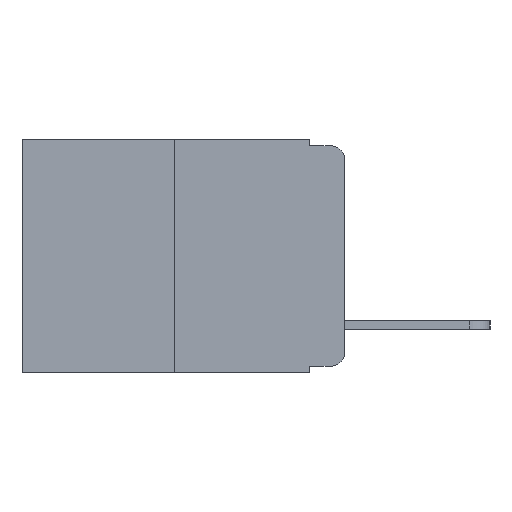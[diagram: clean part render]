
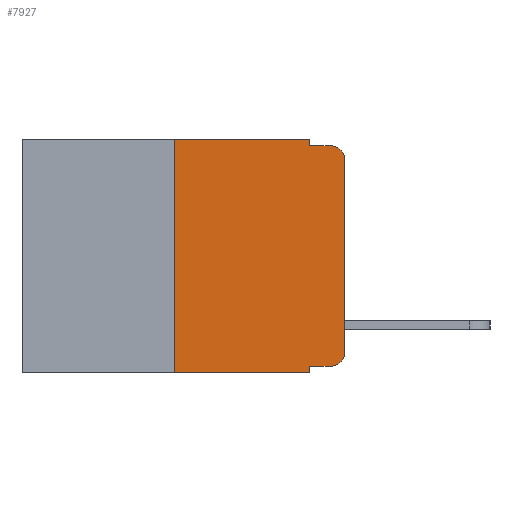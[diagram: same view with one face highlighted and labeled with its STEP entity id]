
A CAD part, left-side view. The second image highlights one B-rep face of the part: STEP entity #7927.
In plain terms, the highlighted planar face has unit normal (-1, 0, 0).
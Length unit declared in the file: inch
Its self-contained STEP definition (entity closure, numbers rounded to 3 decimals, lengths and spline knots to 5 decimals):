
#312 = AXIS2_PLACEMENT_3D ( 'NONE', #5879, #4710, #1290 ) ;
#335 = LINE ( 'NONE', #4685, #9432 ) ;
#344 = ORIENTED_EDGE ( 'NONE', *, *, #2366, .T. ) ;
#508 = DIRECTION ( 'NONE',  ( 0., 0., 1. ) ) ;
#581 = CARTESIAN_POINT ( 'NONE',  ( 0., 0., 0. ) ) ;
#701 = CARTESIAN_POINT ( 'NONE',  ( 0., 0.25, 0. ) ) ;
#743 = ORIENTED_EDGE ( 'NONE', *, *, #3100, .F. ) ;
#872 = ORIENTED_EDGE ( 'NONE', *, *, #5389, .F. ) ;
#877 = VERTEX_POINT ( 'NONE', #701 ) ;
#1074 = VERTEX_POINT ( 'NONE', #11644 ) ;
#1108 = VECTOR ( 'NONE', #1454, 39.37008 ) ;
#1290 = DIRECTION ( 'NONE',  ( 0., 0., -1. ) ) ;
#1291 = ORIENTED_EDGE ( 'NONE', *, *, #4717, .F. ) ;
#1413 = CARTESIAN_POINT ( 'NONE',  ( 0., 0.051, 0. ) ) ;
#1454 = DIRECTION ( 'NONE',  ( 0., 0., -1. ) ) ;
#1519 = VERTEX_POINT ( 'NONE', #2884 ) ;
#1593 = VECTOR ( 'NONE', #2601, 39.37008 ) ;
#1609 = ORIENTED_EDGE ( 'NONE', *, *, #6430, .F. ) ;
#1703 = ORIENTED_EDGE ( 'NONE', *, *, #5988, .T. ) ;
#1829 = LINE ( 'NONE', #10117, #7967 ) ;
#1870 = ORIENTED_EDGE ( 'NONE', *, *, #6578, .F. ) ;
#1884 = ORIENTED_EDGE ( 'NONE', *, *, #7159, .T. ) ;
#1901 = CIRCLE ( 'NONE', #6785, 0.02 ) ;
#1902 = ORIENTED_EDGE ( 'NONE', *, *, #7440, .T. ) ;
#1948 = VERTEX_POINT ( 'NONE', #3599 ) ;
#2026 = DIRECTION ( 'NONE',  ( 1., 0., 0. ) ) ;
#2087 = DIRECTION ( 'NONE',  ( 0., 0., 1. ) ) ;
#2172 = EDGE_CURVE ( 'NONE', #3881, #4770, #8960, .T. ) ;
#2187 = PLANE ( 'NONE',  #7095 ) ;
#2301 = LINE ( 'NONE', #11060, #10924 ) ;
#2366 = EDGE_CURVE ( 'NONE', #4770, #9072, #11750, .T. ) ;
#2601 = DIRECTION ( 'NONE',  ( 0., -1., 0. ) ) ;
#2747 = DIRECTION ( 'NONE',  ( 0., -1., 0. ) ) ;
#2807 = VECTOR ( 'NONE', #508, 39.37008 ) ;
#2884 = CARTESIAN_POINT ( 'NONE',  ( 0., 0.25, -0.343 ) ) ;
#3100 = EDGE_CURVE ( 'NONE', #11806, #9072, #11737, .T. ) ;
#3218 = VERTEX_POINT ( 'NONE', #13384 ) ;
#3599 = CARTESIAN_POINT ( 'NONE',  ( 0., 0.051, 0. ) ) ;
#3881 = VERTEX_POINT ( 'NONE', #10325 ) ;
#4552 = CARTESIAN_POINT ( 'NONE',  ( 0., 0.051, -0.01 ) ) ;
#4596 = DIRECTION ( 'NONE',  ( 0., -1., 0. ) ) ;
#4685 = CARTESIAN_POINT ( 'NONE',  ( 0., 0.473, 0. ) ) ;
#4710 = DIRECTION ( 'NONE',  ( -1., 0., 0. ) ) ;
#4717 = EDGE_CURVE ( 'NONE', #877, #1948, #335, .T. ) ;
#4738 = LINE ( 'NONE', #10747, #7888 ) ;
#4770 = VERTEX_POINT ( 'NONE', #12159 ) ;
#4798 = EDGE_LOOP ( 'NONE', ( #12902, #344, #743, #872, #1291, #1609, #1703, #1870, #1884, #1902 ) ) ;
#4804 = VERTEX_POINT ( 'NONE', #7604 ) ;
#4945 = LINE ( 'NONE', #5333, #1593 ) ;
#5062 = CARTESIAN_POINT ( 'NONE',  ( 0., 0.473, 0. ) ) ;
#5333 = CARTESIAN_POINT ( 'NONE',  ( 0., 0.473, -0.343 ) ) ;
#5389 = EDGE_CURVE ( 'NONE', #1948, #11806, #1829, .T. ) ;
#5643 = DIRECTION ( 'NONE',  ( 0., 0., -1. ) ) ;
#5701 = DIRECTION ( 'NONE',  ( -1., 0., 0. ) ) ;
#5879 = CARTESIAN_POINT ( 'NONE',  ( 0., 0.02, -0.03 ) ) ;
#5988 = EDGE_CURVE ( 'NONE', #1519, #1074, #4945, .T. ) ;
#6430 = EDGE_CURVE ( 'NONE', #1519, #877, #4738, .T. ) ;
#6578 = EDGE_CURVE ( 'NONE', #4804, #1074, #10949, .T. ) ;
#6785 = AXIS2_PLACEMENT_3D ( 'NONE', #8881, #5701, #5643 ) ;
#7009 = DIRECTION ( 'NONE',  ( 0., 0., -1. ) ) ;
#7095 = AXIS2_PLACEMENT_3D ( 'NONE', #5062, #2026, #7009 ) ;
#7159 = EDGE_CURVE ( 'NONE', #4804, #3218, #2301, .T. ) ;
#7440 = EDGE_CURVE ( 'NONE', #3218, #3881, #1901, .T. ) ;
#7604 = CARTESIAN_POINT ( 'NONE',  ( 0., 0.051, -0.333 ) ) ;
#7888 = VECTOR ( 'NONE', #2087, 39.37008 ) ;
#7927 = ADVANCED_FACE ( 'NONE', ( #8220 ), #2187, .F. ) ;
#7967 = VECTOR ( 'NONE', #10753, 39.37008 ) ;
#8220 = FACE_OUTER_BOUND ( 'NONE', #4798, .T. ) ;
#8881 = CARTESIAN_POINT ( 'NONE',  ( 0., 0.02, -0.313 ) ) ;
#8960 = LINE ( 'NONE', #581, #2807 ) ;
#9072 = VERTEX_POINT ( 'NONE', #13960 ) ;
#9126 = VECTOR ( 'NONE', #4596, 39.37008 ) ;
#9432 = VECTOR ( 'NONE', #10571, 39.37008 ) ;
#10117 = CARTESIAN_POINT ( 'NONE',  ( 0., 0.051, 0. ) ) ;
#10325 = CARTESIAN_POINT ( 'NONE',  ( 0., 0., -0.313 ) ) ;
#10571 = DIRECTION ( 'NONE',  ( 0., -1., 0. ) ) ;
#10747 = CARTESIAN_POINT ( 'NONE',  ( 0., 0.25, 0. ) ) ;
#10753 = DIRECTION ( 'NONE',  ( 0., 0., -1. ) ) ;
#10924 = VECTOR ( 'NONE', #2747, 39.37008 ) ;
#10949 = LINE ( 'NONE', #1413, #1108 ) ;
#11060 = CARTESIAN_POINT ( 'NONE',  ( 0., 0.051, -0.333 ) ) ;
#11644 = CARTESIAN_POINT ( 'NONE',  ( 0., 0.051, -0.343 ) ) ;
#11737 = LINE ( 'NONE', #4552, #9126 ) ;
#11750 = CIRCLE ( 'NONE', #312, 0.02 ) ;
#11806 = VERTEX_POINT ( 'NONE', #12355 ) ;
#12159 = CARTESIAN_POINT ( 'NONE',  ( 0., 0., -0.03 ) ) ;
#12355 = CARTESIAN_POINT ( 'NONE',  ( 0., 0.051, -0.01 ) ) ;
#12902 = ORIENTED_EDGE ( 'NONE', *, *, #2172, .T. ) ;
#13384 = CARTESIAN_POINT ( 'NONE',  ( 0., 0.02, -0.333 ) ) ;
#13960 = CARTESIAN_POINT ( 'NONE',  ( 0., 0.02, -0.01 ) ) ;
